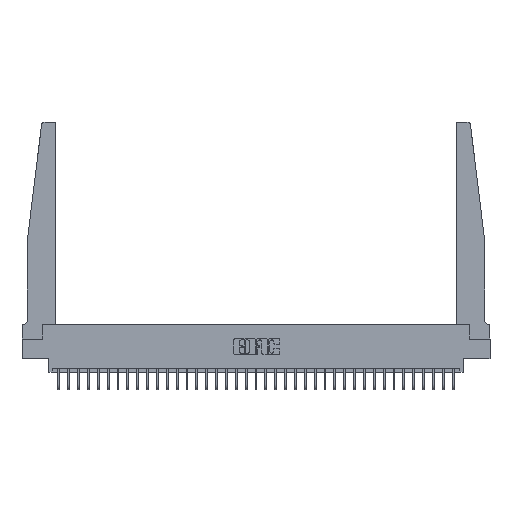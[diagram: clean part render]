
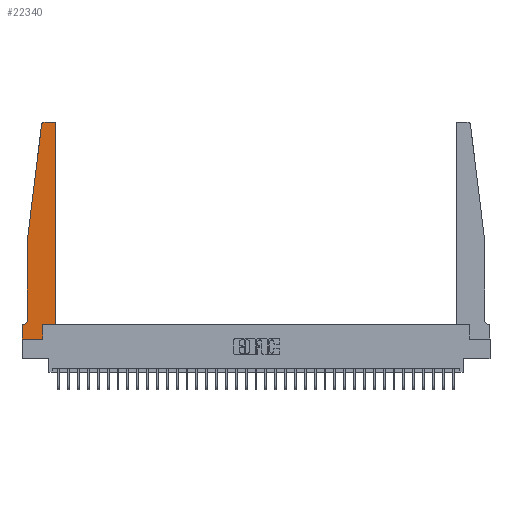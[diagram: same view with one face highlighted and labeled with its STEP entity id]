
A CAD part, top view. The second image highlights one B-rep face of the part: STEP entity #22340.
In plain terms, the highlighted planar face has unit normal (0, 0, 1).
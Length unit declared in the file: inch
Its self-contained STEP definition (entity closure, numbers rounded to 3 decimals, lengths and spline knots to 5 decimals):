
#631 = CARTESIAN_POINT ( 'NONE',  ( 0.2605, 0., 0.37 ) ) ;
#1057 = ORIENTED_EDGE ( 'NONE', *, *, #20833, .T. ) ;
#1240 = VECTOR ( 'NONE', #26174, 39.37008 ) ;
#1458 = EDGE_CURVE ( 'NONE', #29111, #11279, #11933, .T. ) ;
#1704 = VECTOR ( 'NONE', #16957, 39.37008 ) ;
#1793 = ORIENTED_EDGE ( 'NONE', *, *, #33346, .T. ) ;
#2476 = CARTESIAN_POINT ( 'NONE',  ( 0.425, 0.18, 0.37 ) ) ;
#2768 = VERTEX_POINT ( 'NONE', #15546 ) ;
#3446 = ORIENTED_EDGE ( 'NONE', *, *, #1458, .T. ) ;
#3525 = DIRECTION ( 'NONE',  ( 1., 0., 0. ) ) ;
#3567 = CARTESIAN_POINT ( 'NONE',  ( 0.2605, 0.18, 0.37 ) ) ;
#4546 = ORIENTED_EDGE ( 'NONE', *, *, #27328, .T. ) ;
#4770 = VERTEX_POINT ( 'NONE', #20811 ) ;
#4856 = DIRECTION ( 'NONE',  ( 1., 0., 0. ) ) ;
#4964 = DIRECTION ( 'NONE',  ( 0., 0., -1. ) ) ;
#5266 = CIRCLE ( 'NONE', #32265, 0.03 ) ;
#5347 = VERTEX_POINT ( 'NONE', #20614 ) ;
#6129 = CARTESIAN_POINT ( 'NONE',  ( 0., 0.1875, 0.37 ) ) ;
#7602 = CARTESIAN_POINT ( 'NONE',  ( 0., 0., 0.37 ) ) ;
#8729 = VERTEX_POINT ( 'NONE', #19539 ) ;
#9065 = PLANE ( 'NONE',  #13996 ) ;
#9132 = VECTOR ( 'NONE', #10742, 39.37008 ) ;
#9895 = LINE ( 'NONE', #20237, #31014 ) ;
#10245 = CARTESIAN_POINT ( 'NONE',  ( 0.065, 1.25, 0.37 ) ) ;
#10628 = CARTESIAN_POINT ( 'NONE',  ( 0.015, 0.1875, 0.37 ) ) ;
#10742 = DIRECTION ( 'NONE',  ( 1., 0., 0. ) ) ;
#11249 = CARTESIAN_POINT ( 'NONE',  ( 0.425, 0.18, 0.37 ) ) ;
#11279 = VERTEX_POINT ( 'NONE', #21846 ) ;
#11339 = CIRCLE ( 'NONE', #30608, 0.05 ) ;
#11667 = LINE ( 'NONE', #32876, #30778 ) ;
#11933 = LINE ( 'NONE', #22446, #19365 ) ;
#12548 = DIRECTION ( 'NONE',  ( -1., 0., 0. ) ) ;
#12965 = VERTEX_POINT ( 'NONE', #10628 ) ;
#13310 = LINE ( 'NONE', #2476, #9132 ) ;
#13996 = AXIS2_PLACEMENT_3D ( 'NONE', #6129, #24595, #16649 ) ;
#14404 = VECTOR ( 'NONE', #4856, 39.37008 ) ;
#14511 = DIRECTION ( 'NONE',  ( 0., 1., 0. ) ) ;
#14772 = CARTESIAN_POINT ( 'NONE',  ( 0.065, 0.2375, 0.37 ) ) ;
#15226 = DIRECTION ( 'NONE',  ( 0., 0., 1. ) ) ;
#15283 = ORIENTED_EDGE ( 'NONE', *, *, #20014, .T. ) ;
#15321 = CARTESIAN_POINT ( 'NONE',  ( 0., 0., 0.37 ) ) ;
#15495 = ORIENTED_EDGE ( 'NONE', *, *, #16716, .T. ) ;
#15546 = CARTESIAN_POINT ( 'NONE',  ( 0.395, 2.75, 0.37 ) ) ;
#15655 = LINE ( 'NONE', #15321, #1240 ) ;
#15867 = ORIENTED_EDGE ( 'NONE', *, *, #20864, .T. ) ;
#15996 = VERTEX_POINT ( 'NONE', #26213 ) ;
#16024 = LINE ( 'NONE', #7602, #14404 ) ;
#16649 = DIRECTION ( 'NONE',  ( 1., 0., 0. ) ) ;
#16716 = EDGE_CURVE ( 'NONE', #32750, #5347, #33025, .T. ) ;
#16781 = LINE ( 'NONE', #32815, #1704 ) ;
#16957 = DIRECTION ( 'NONE',  ( -1., 0., 0. ) ) ;
#17433 = CIRCLE ( 'NONE', #28471, 0.03 ) ;
#18566 = ORIENTED_EDGE ( 'NONE', *, *, #30056, .T. ) ;
#19195 = VERTEX_POINT ( 'NONE', #33714 ) ;
#19365 = VECTOR ( 'NONE', #14511, 39.37008 ) ;
#19539 = CARTESIAN_POINT ( 'NONE',  ( 0., 0.1875, 0.37 ) ) ;
#19560 = EDGE_CURVE ( 'NONE', #19195, #32750, #16024, .T. ) ;
#19598 = DIRECTION ( 'NONE',  ( 0., 1., 0. ) ) ;
#20014 = EDGE_CURVE ( 'NONE', #8729, #19195, #15655, .T. ) ;
#20237 = CARTESIAN_POINT ( 'NONE',  ( 0.065, 0.1875, 0.37 ) ) ;
#20614 = CARTESIAN_POINT ( 'NONE',  ( 0.2605, 0.18, 0.37 ) ) ;
#20811 = CARTESIAN_POINT ( 'NONE',  ( 0.27653, 2.75, 0.37 ) ) ;
#20833 = EDGE_CURVE ( 'NONE', #21225, #32717, #31105, .T. ) ;
#20864 = EDGE_CURVE ( 'NONE', #12965, #8729, #9895, .T. ) ;
#21225 = VERTEX_POINT ( 'NONE', #24533 ) ;
#21846 = CARTESIAN_POINT ( 'NONE',  ( 0.425, 2.72, 0.37 ) ) ;
#22340 = ADVANCED_FACE ( 'NONE', ( #27507 ), #9065, .T. ) ;
#22446 = CARTESIAN_POINT ( 'NONE',  ( 0.425, 0.18, 0.37 ) ) ;
#22468 = DIRECTION ( 'NONE',  ( 1., 0., 0. ) ) ;
#22777 = EDGE_LOOP ( 'NONE', ( #1793, #4546, #18566, #1057, #27543, #15867, #15283, #28033, #15495, #24623, #3446, #32666 ) ) ;
#22849 = DIRECTION ( 'NONE',  ( -0.122, -0.992, 0. ) ) ;
#24294 = EDGE_CURVE ( 'NONE', #11279, #2768, #5266, .T. ) ;
#24420 = EDGE_CURVE ( 'NONE', #5347, #29111, #13310, .T. ) ;
#24533 = CARTESIAN_POINT ( 'NONE',  ( 0.065, 1.25, 0.37 ) ) ;
#24595 = DIRECTION ( 'NONE',  ( 0., 0., 1. ) ) ;
#24623 = ORIENTED_EDGE ( 'NONE', *, *, #24420, .T. ) ;
#24726 = DIRECTION ( 'NONE',  ( 0., 0., 1. ) ) ;
#25227 = CARTESIAN_POINT ( 'NONE',  ( 0.395, 2.72, 0.37 ) ) ;
#26174 = DIRECTION ( 'NONE',  ( 0., -1., 0. ) ) ;
#26213 = CARTESIAN_POINT ( 'NONE',  ( 0.24675, 2.72367, 0.37 ) ) ;
#26588 = EDGE_CURVE ( 'NONE', #32717, #12965, #11339, .T. ) ;
#27301 = DIRECTION ( 'NONE',  ( -1., 0., 0. ) ) ;
#27328 = EDGE_CURVE ( 'NONE', #4770, #15996, #17433, .T. ) ;
#27507 = FACE_OUTER_BOUND ( 'NONE', #22777, .T. ) ;
#27543 = ORIENTED_EDGE ( 'NONE', *, *, #26588, .T. ) ;
#28033 = ORIENTED_EDGE ( 'NONE', *, *, #19560, .T. ) ;
#28332 = DIRECTION ( 'NONE',  ( 0., -1., 0. ) ) ;
#28471 = AXIS2_PLACEMENT_3D ( 'NONE', #31965, #24726, #3525 ) ;
#29111 = VERTEX_POINT ( 'NONE', #11249 ) ;
#29332 = VECTOR ( 'NONE', #28332, 39.37008 ) ;
#30056 = EDGE_CURVE ( 'NONE', #15996, #21225, #11667, .T. ) ;
#30608 = AXIS2_PLACEMENT_3D ( 'NONE', #33578, #4964, #12548 ) ;
#30778 = VECTOR ( 'NONE', #22849, 39.37008 ) ;
#30961 = VECTOR ( 'NONE', #19598, 39.37008 ) ;
#31014 = VECTOR ( 'NONE', #27301, 39.37008 ) ;
#31105 = LINE ( 'NONE', #10245, #29332 ) ;
#31965 = CARTESIAN_POINT ( 'NONE',  ( 0.27653, 2.72, 0.37 ) ) ;
#32265 = AXIS2_PLACEMENT_3D ( 'NONE', #25227, #15226, #22468 ) ;
#32666 = ORIENTED_EDGE ( 'NONE', *, *, #24294, .T. ) ;
#32717 = VERTEX_POINT ( 'NONE', #14772 ) ;
#32750 = VERTEX_POINT ( 'NONE', #631 ) ;
#32815 = CARTESIAN_POINT ( 'NONE',  ( 0.25, 2.75, 0.37 ) ) ;
#32876 = CARTESIAN_POINT ( 'NONE',  ( 0.065, 1.25, 0.37 ) ) ;
#33025 = LINE ( 'NONE', #3567, #30961 ) ;
#33346 = EDGE_CURVE ( 'NONE', #2768, #4770, #16781, .T. ) ;
#33578 = CARTESIAN_POINT ( 'NONE',  ( 0.015, 0.2375, 0.37 ) ) ;
#33714 = CARTESIAN_POINT ( 'NONE',  ( 0., 0., 0.37 ) ) ;
